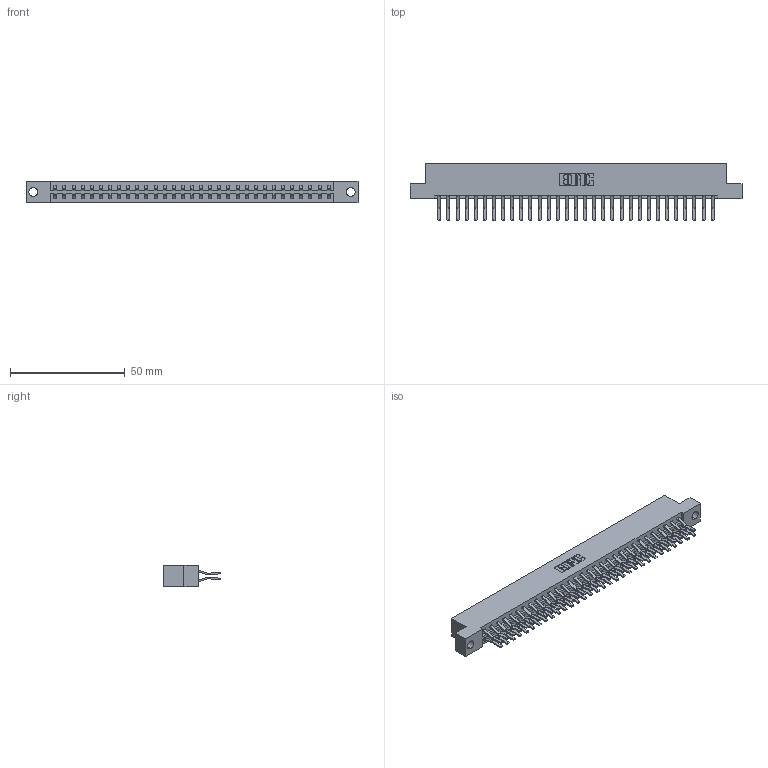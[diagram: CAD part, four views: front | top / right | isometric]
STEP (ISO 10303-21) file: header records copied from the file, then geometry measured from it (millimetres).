
FILE_DESCRIPTION (( 'STEP AP203' ), '1' );
FILE_NAME ('833-062-560-204.STEP', '2020-06-05T06:28:22', ( '' ), ( '' ), 'SwSTEP 2.0', 'SolidWorks 2020', '' );
FILE_SCHEMA (( 'CONFIG_CONTROL_DESIGN' ));
Length unit declared in the file: inch
Products named in the file (3): 833-062-560-204; 833 Part_Flush - .156 Dia - TH; 345-292-001_560 Tail
Assembly tree (63 placements, depth 2):
  833-062-560-204
    833 Part_Flush - .156 Dia - TH
    345-292-001_560 Tail  x62
Bounding box: 144.37 x 24.78 x 9.4 mm (x, y, z)
Volume: 14955.4 mm3; surface area: 18521.5 mm2
Topology: 63 solids, 63 shells, 3462 faces, 10293 edges, 6778 vertices
Faces by surface type: plane 2302, cylinder 1160
Entity records: 21457 total; most frequent: CARTESIAN_POINT 3570, ORIENTED_EDGE 3506, DIRECTION 3073, EDGE_CURVE 1753, LINE 1621, VECTOR 1621, VERTEX_POINT 1166, AXIS2_PLACEMENT_3D 726
